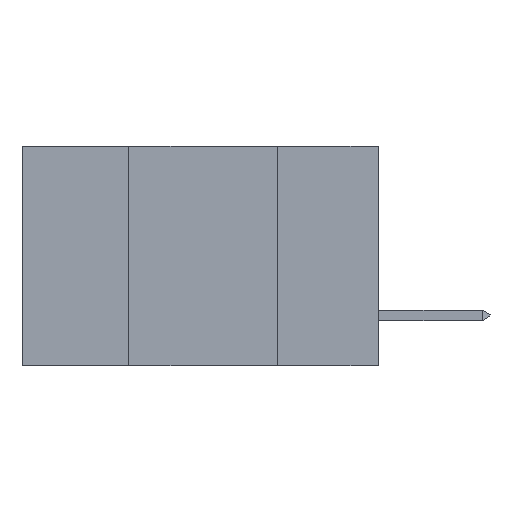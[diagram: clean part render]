
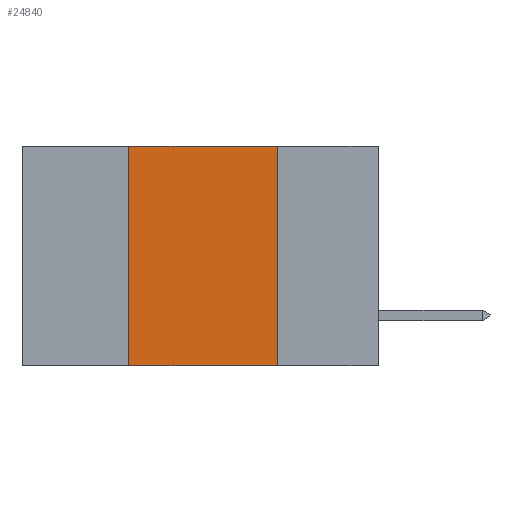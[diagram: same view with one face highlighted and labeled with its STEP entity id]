
A CAD part, left-side view. The second image highlights one B-rep face of the part: STEP entity #24840.
In plain terms, the highlighted planar face has unit normal (-1, 0, 0).
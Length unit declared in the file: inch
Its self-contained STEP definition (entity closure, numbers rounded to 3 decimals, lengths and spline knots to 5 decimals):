
#225 = CARTESIAN_POINT ( 'NONE',  ( 0., 0.17, -0.37 ) ) ;
#395 = LINE ( 'NONE', #4626, #5769 ) ;
#1366 = EDGE_CURVE ( 'NONE', #6158, #8081, #395, .T. ) ;
#3090 = DIRECTION ( 'NONE',  ( 0., 0., -1. ) ) ;
#4626 = CARTESIAN_POINT ( 'NONE',  ( 0., 0.42, -0.37 ) ) ;
#5272 = CARTESIAN_POINT ( 'NONE',  ( 0., 0.6, 0. ) ) ;
#5439 = VECTOR ( 'NONE', #3090, 39.37008 ) ;
#5705 = LINE ( 'NONE', #13439, #8603 ) ;
#5769 = VECTOR ( 'NONE', #18087, 39.37008 ) ;
#6158 = VERTEX_POINT ( 'NONE', #24811 ) ;
#6691 = AXIS2_PLACEMENT_3D ( 'NONE', #5272, #13021, #16569 ) ;
#6920 = LINE ( 'NONE', #8942, #7844 ) ;
#7844 = VECTOR ( 'NONE', #18434, 39.37008 ) ;
#8081 = VERTEX_POINT ( 'NONE', #15185 ) ;
#8603 = VECTOR ( 'NONE', #19274, 39.37008 ) ;
#8942 = CARTESIAN_POINT ( 'NONE',  ( 0., 0.6, 0. ) ) ;
#9124 = FACE_OUTER_BOUND ( 'NONE', #13856, .T. ) ;
#11364 = CARTESIAN_POINT ( 'NONE',  ( 0., 0.17, 0. ) ) ;
#12033 = EDGE_CURVE ( 'NONE', #17449, #19863, #14755, .T. ) ;
#12779 = ORIENTED_EDGE ( 'NONE', *, *, #1366, .F. ) ;
#13021 = DIRECTION ( 'NONE',  ( 1., 0., 0. ) ) ;
#13439 = CARTESIAN_POINT ( 'NONE',  ( 0., 0.6, -0.37 ) ) ;
#13856 = EDGE_LOOP ( 'NONE', ( #19220, #17189, #12779, #21330 ) ) ;
#14755 = LINE ( 'NONE', #22540, #5439 ) ;
#15185 = CARTESIAN_POINT ( 'NONE',  ( 0., 0.42, 0. ) ) ;
#16569 = DIRECTION ( 'NONE',  ( 0., 0., -1. ) ) ;
#16819 = PLANE ( 'NONE',  #6691 ) ;
#17189 = ORIENTED_EDGE ( 'NONE', *, *, #20780, .F. ) ;
#17449 = VERTEX_POINT ( 'NONE', #11364 ) ;
#18087 = DIRECTION ( 'NONE',  ( 0., 0., 1. ) ) ;
#18434 = DIRECTION ( 'NONE',  ( 0., -1., 0. ) ) ;
#19220 = ORIENTED_EDGE ( 'NONE', *, *, #12033, .F. ) ;
#19274 = DIRECTION ( 'NONE',  ( 0., -1., 0. ) ) ;
#19863 = VERTEX_POINT ( 'NONE', #225 ) ;
#20203 = EDGE_CURVE ( 'NONE', #6158, #19863, #5705, .T. ) ;
#20780 = EDGE_CURVE ( 'NONE', #8081, #17449, #6920, .T. ) ;
#21330 = ORIENTED_EDGE ( 'NONE', *, *, #20203, .T. ) ;
#22540 = CARTESIAN_POINT ( 'NONE',  ( 0., 0.17, -0.37 ) ) ;
#24811 = CARTESIAN_POINT ( 'NONE',  ( 0., 0.42, -0.37 ) ) ;
#24840 = ADVANCED_FACE ( 'NONE', ( #9124 ), #16819, .F. ) ;
